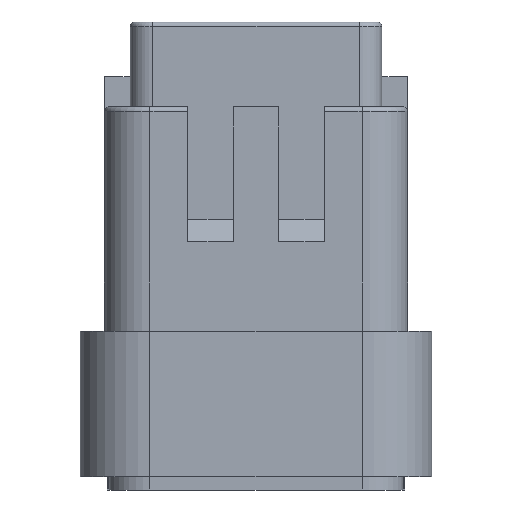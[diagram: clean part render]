
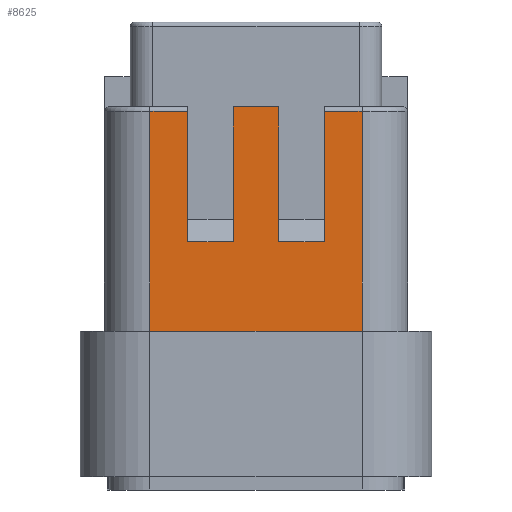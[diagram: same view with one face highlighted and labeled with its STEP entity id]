
A CAD part, front view. The second image highlights one B-rep face of the part: STEP entity #8625.
In plain terms, the highlighted planar face has unit normal (0, -1, 0).
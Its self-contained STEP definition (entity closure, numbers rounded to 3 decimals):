
#511 = DIRECTION ( 'NONE',  ( -1., 0., 0. ) ) ;
#704 = CARTESIAN_POINT ( 'NONE',  ( 6.4, -0.75, -6.4 ) ) ;
#890 = CARTESIAN_POINT ( 'NONE',  ( 1.9, -0.75, -6.4 ) ) ;
#1022 = VECTOR ( 'NONE', #10058, 1000. ) ;
#1046 = EDGE_CURVE ( 'NONE', #3609, #8029, #2321, .T. ) ;
#1068 = VECTOR ( 'NONE', #6966, 1000. ) ;
#1113 = CARTESIAN_POINT ( 'NONE',  ( 7.65, -0.75, -10.2 ) ) ;
#1122 = VECTOR ( 'NONE', #511, 1000. ) ;
#1203 = CARTESIAN_POINT ( 'NONE',  ( 4.9, -0.75, -7.25 ) ) ;
#1259 = VECTOR ( 'NONE', #6394, 1000. ) ;
#1613 = CARTESIAN_POINT ( 'NONE',  ( 7.65, -0.75, -10.2 ) ) ;
#1816 = CARTESIAN_POINT ( 'NONE',  ( 3.4, -0.75, -2.8 ) ) ;
#1890 = CARTESIAN_POINT ( 'NONE',  ( 6.4, -0.75, -2.95 ) ) ;
#2102 = CARTESIAN_POINT ( 'NONE',  ( 4.9, -0.75, -7.25 ) ) ;
#2204 = CARTESIAN_POINT ( 'NONE',  ( 0.65, -0.75, -2.95 ) ) ;
#2321 = LINE ( 'NONE', #9393, #1122 ) ;
#2378 = CARTESIAN_POINT ( 'NONE',  ( 6.4, -0.75, -2.95 ) ) ;
#2380 = VERTEX_POINT ( 'NONE', #1203 ) ;
#2598 = ORIENTED_EDGE ( 'NONE', *, *, #3139, .T. ) ;
#2645 = VERTEX_POINT ( 'NONE', #12206 ) ;
#3122 = EDGE_CURVE ( 'NONE', #10572, #4162, #11100, .T. ) ;
#3139 = EDGE_CURVE ( 'NONE', #2645, #7267, #7072, .T. ) ;
#3229 = CARTESIAN_POINT ( 'NONE',  ( 1.9, -0.75, -7.25 ) ) ;
#3282 = PLANE ( 'NONE',  #12616 ) ;
#3366 = ORIENTED_EDGE ( 'NONE', *, *, #10464, .T. ) ;
#3402 = EDGE_CURVE ( 'NONE', #9063, #4146, #10697, .T. ) ;
#3478 = VECTOR ( 'NONE', #8364, 1000. ) ;
#3609 = VERTEX_POINT ( 'NONE', #4004 ) ;
#3778 = LINE ( 'NONE', #6829, #7675 ) ;
#3961 = ORIENTED_EDGE ( 'NONE', *, *, #3402, .F. ) ;
#4004 = CARTESIAN_POINT ( 'NONE',  ( 3.4, -0.75, -7.25 ) ) ;
#4146 = VERTEX_POINT ( 'NONE', #1890 ) ;
#4162 = VERTEX_POINT ( 'NONE', #5971 ) ;
#4240 = CARTESIAN_POINT ( 'NONE',  ( 6.4, -0.75, -7.25 ) ) ;
#4354 = EDGE_CURVE ( 'NONE', #12084, #7853, #11035, .T. ) ;
#4708 = CARTESIAN_POINT ( 'NONE',  ( 4.9, -0.75, -2.8 ) ) ;
#5127 = DIRECTION ( 'NONE',  ( -1., 0., 0. ) ) ;
#5232 = EDGE_CURVE ( 'NONE', #7743, #4162, #5407, .T. ) ;
#5407 = LINE ( 'NONE', #6374, #11645 ) ;
#5486 = ORIENTED_EDGE ( 'NONE', *, *, #8045, .F. ) ;
#5633 = DIRECTION ( 'NONE',  ( 0., 0., 1. ) ) ;
#5971 = CARTESIAN_POINT ( 'NONE',  ( 0.65, -0.75, -2.95 ) ) ;
#6104 = CARTESIAN_POINT ( 'NONE',  ( 7.65, -0.75, -2.8 ) ) ;
#6374 = CARTESIAN_POINT ( 'NONE',  ( 0.65, -0.75, -10.2 ) ) ;
#6394 = DIRECTION ( 'NONE',  ( -1., 0., 0. ) ) ;
#6829 = CARTESIAN_POINT ( 'NONE',  ( 3.4, -0.75, -6.4 ) ) ;
#6848 = LINE ( 'NONE', #8084, #11806 ) ;
#6903 = ORIENTED_EDGE ( 'NONE', *, *, #5232, .F. ) ;
#6922 = VECTOR ( 'NONE', #5127, 1000. ) ;
#6966 = DIRECTION ( 'NONE',  ( -1., 0., 0. ) ) ;
#7072 = LINE ( 'NONE', #1113, #12487 ) ;
#7196 = EDGE_LOOP ( 'NONE', ( #2598, #9331, #3961, #3366, #8087, #8221, #10993, #12511, #7326, #7522, #6903, #5486 ) ) ;
#7251 = CARTESIAN_POINT ( 'NONE',  ( 7.65, -0.75, -10.2 ) ) ;
#7267 = VERTEX_POINT ( 'NONE', #11731 ) ;
#7326 = ORIENTED_EDGE ( 'NONE', *, *, #11405, .T. ) ;
#7383 = LINE ( 'NONE', #2378, #1259 ) ;
#7522 = ORIENTED_EDGE ( 'NONE', *, *, #3122, .T. ) ;
#7526 = CARTESIAN_POINT ( 'NONE',  ( 0.65, -0.75, -10.2 ) ) ;
#7675 = VECTOR ( 'NONE', #7754, 1000. ) ;
#7743 = VERTEX_POINT ( 'NONE', #7526 ) ;
#7754 = DIRECTION ( 'NONE',  ( 0., 0., 1. ) ) ;
#7853 = VERTEX_POINT ( 'NONE', #1816 ) ;
#8029 = VERTEX_POINT ( 'NONE', #3229 ) ;
#8045 = EDGE_CURVE ( 'NONE', #2645, #7743, #11402, .T. ) ;
#8084 = CARTESIAN_POINT ( 'NONE',  ( 4.9, -0.75, -6.4 ) ) ;
#8087 = ORIENTED_EDGE ( 'NONE', *, *, #8946, .T. ) ;
#8221 = ORIENTED_EDGE ( 'NONE', *, *, #4354, .T. ) ;
#8364 = DIRECTION ( 'NONE',  ( -1., 0., 0. ) ) ;
#8541 = VECTOR ( 'NONE', #5633, 1000. ) ;
#8625 = ADVANCED_FACE ( 'NONE', ( #9199 ), #3282, .F. ) ;
#8924 = DIRECTION ( 'NONE',  ( 0., 0., 1. ) ) ;
#8946 = EDGE_CURVE ( 'NONE', #2380, #12084, #6848, .T. ) ;
#9051 = DIRECTION ( 'NONE',  ( 0., 0., 1. ) ) ;
#9063 = VERTEX_POINT ( 'NONE', #4240 ) ;
#9199 = FACE_OUTER_BOUND ( 'NONE', #7196, .T. ) ;
#9331 = ORIENTED_EDGE ( 'NONE', *, *, #9872, .T. ) ;
#9339 = EDGE_CURVE ( 'NONE', #3609, #7853, #3778, .T. ) ;
#9393 = CARTESIAN_POINT ( 'NONE',  ( 1.9, -0.75, -7.25 ) ) ;
#9759 = LINE ( 'NONE', #2102, #1068 ) ;
#9872 = EDGE_CURVE ( 'NONE', #7267, #4146, #7383, .T. ) ;
#10058 = DIRECTION ( 'NONE',  ( -1., 0., 0. ) ) ;
#10270 = CARTESIAN_POINT ( 'NONE',  ( 1.9, -0.75, -2.95 ) ) ;
#10339 = DIRECTION ( 'NONE',  ( 0., 0., 1. ) ) ;
#10464 = EDGE_CURVE ( 'NONE', #9063, #2380, #9759, .T. ) ;
#10572 = VERTEX_POINT ( 'NONE', #10270 ) ;
#10697 = LINE ( 'NONE', #704, #8541 ) ;
#10993 = ORIENTED_EDGE ( 'NONE', *, *, #9339, .F. ) ;
#11035 = LINE ( 'NONE', #6104, #1022 ) ;
#11100 = LINE ( 'NONE', #2204, #6922 ) ;
#11140 = VECTOR ( 'NONE', #8924, 1000. ) ;
#11209 = DIRECTION ( 'NONE',  ( -1., 0., 0. ) ) ;
#11402 = LINE ( 'NONE', #1613, #3478 ) ;
#11405 = EDGE_CURVE ( 'NONE', #8029, #10572, #11913, .T. ) ;
#11645 = VECTOR ( 'NONE', #10339, 1000. ) ;
#11731 = CARTESIAN_POINT ( 'NONE',  ( 7.65, -0.75, -2.95 ) ) ;
#11806 = VECTOR ( 'NONE', #9051, 1000. ) ;
#11913 = LINE ( 'NONE', #890, #11140 ) ;
#11941 = DIRECTION ( 'NONE',  ( 0., 0., 1. ) ) ;
#12084 = VERTEX_POINT ( 'NONE', #4708 ) ;
#12206 = CARTESIAN_POINT ( 'NONE',  ( 7.65, -0.75, -10.2 ) ) ;
#12319 = DIRECTION ( 'NONE',  ( 0., 1., 0. ) ) ;
#12487 = VECTOR ( 'NONE', #11941, 1000. ) ;
#12511 = ORIENTED_EDGE ( 'NONE', *, *, #1046, .T. ) ;
#12616 = AXIS2_PLACEMENT_3D ( 'NONE', #7251, #12319, #11209 ) ;
